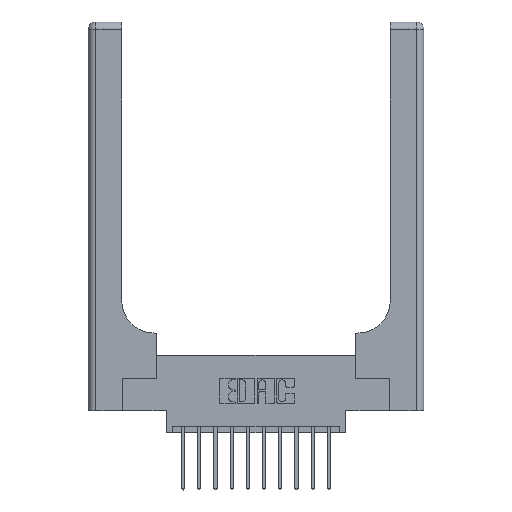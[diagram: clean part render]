
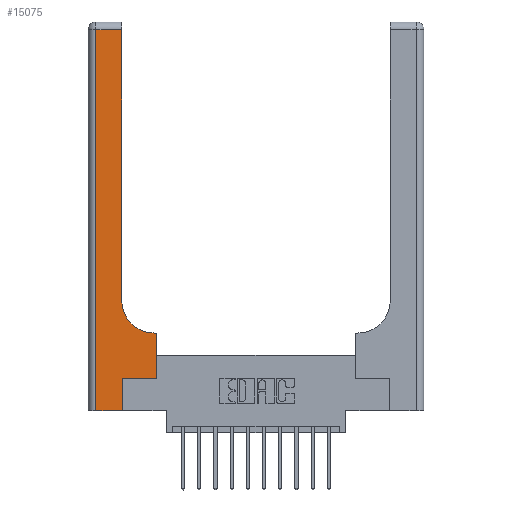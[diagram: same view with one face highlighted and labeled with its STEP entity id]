
A CAD part, top view. The second image highlights one B-rep face of the part: STEP entity #15075.
In plain terms, the highlighted planar face has unit normal (0, 0, 1).
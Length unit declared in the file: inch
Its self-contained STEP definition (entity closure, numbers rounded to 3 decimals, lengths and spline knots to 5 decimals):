
#54 = EDGE_CURVE ( 'NONE', #11182, #409, #9002, .T. ) ;
#239 = DIRECTION ( 'NONE',  ( 0., 0., -1. ) ) ;
#258 = DIRECTION ( 'NONE',  ( 0., 1., 0. ) ) ;
#409 = VERTEX_POINT ( 'NONE', #15262 ) ;
#423 = EDGE_CURVE ( 'NONE', #1495, #7632, #7598, .T. ) ;
#879 = DIRECTION ( 'NONE',  ( -1., 0., 0. ) ) ;
#1193 = ORIENTED_EDGE ( 'NONE', *, *, #54, .T. ) ;
#1268 = LINE ( 'NONE', #7843, #14576 ) ;
#1495 = VERTEX_POINT ( 'NONE', #8806 ) ;
#1577 = CARTESIAN_POINT ( 'NONE',  ( 0.26, 3., 0.37 ) ) ;
#1622 = DIRECTION ( 'NONE',  ( 0., -1., 0. ) ) ;
#1804 = DIRECTION ( 'NONE',  ( 1., 0., 0. ) ) ;
#2093 = ORIENTED_EDGE ( 'NONE', *, *, #2830, .T. ) ;
#2153 = CARTESIAN_POINT ( 'NONE',  ( 0., 2.94, 0.37 ) ) ;
#2456 = EDGE_LOOP ( 'NONE', ( #12871, #12136, #6369, #4838, #4947, #2093, #2734, #1193, #13378 ) ) ;
#2734 = ORIENTED_EDGE ( 'NONE', *, *, #3348, .T. ) ;
#2746 = EDGE_CURVE ( 'NONE', #15318, #7378, #5762, .T. ) ;
#2830 = EDGE_CURVE ( 'NONE', #7632, #5285, #5391, .T. ) ;
#2874 = CARTESIAN_POINT ( 'NONE',  ( 0.06, 3., 0.37 ) ) ;
#3275 = CARTESIAN_POINT ( 'NONE',  ( 0.265, 0.25, 0.37 ) ) ;
#3348 = EDGE_CURVE ( 'NONE', #5285, #11182, #1268, .T. ) ;
#3656 = EDGE_CURVE ( 'NONE', #14289, #15318, #6920, .T. ) ;
#4657 = VECTOR ( 'NONE', #258, 39.37008 ) ;
#4838 = ORIENTED_EDGE ( 'NONE', *, *, #12543, .T. ) ;
#4947 = ORIENTED_EDGE ( 'NONE', *, *, #423, .T. ) ;
#5273 = VECTOR ( 'NONE', #7014, 39.37008 ) ;
#5285 = VERTEX_POINT ( 'NONE', #15860 ) ;
#5391 = LINE ( 'NONE', #11786, #7926 ) ;
#5394 = CARTESIAN_POINT ( 'NONE',  ( 0., 0., 0.37 ) ) ;
#5567 = VECTOR ( 'NONE', #12917, 39.37008 ) ;
#5762 = LINE ( 'NONE', #2874, #12457 ) ;
#5952 = LINE ( 'NONE', #5394, #5567 ) ;
#6024 = CARTESIAN_POINT ( 'NONE',  ( 0.528, 0.6, 0.37 ) ) ;
#6028 = CARTESIAN_POINT ( 'NONE',  ( 0.26, 0.85, 0.37 ) ) ;
#6369 = ORIENTED_EDGE ( 'NONE', *, *, #2746, .T. ) ;
#6869 = EDGE_CURVE ( 'NONE', #12926, #14289, #14419, .T. ) ;
#6901 = CARTESIAN_POINT ( 'NONE',  ( 0.06, 2.94, 0.37 ) ) ;
#6920 = LINE ( 'NONE', #2153, #9893 ) ;
#7014 = DIRECTION ( 'NONE',  ( -1., 0., 0. ) ) ;
#7131 = CARTESIAN_POINT ( 'NONE',  ( 0.51, 0.85, 0.37 ) ) ;
#7142 = EDGE_CURVE ( 'NONE', #409, #12926, #13857, .T. ) ;
#7378 = VERTEX_POINT ( 'NONE', #10061 ) ;
#7598 = LINE ( 'NONE', #12763, #4657 ) ;
#7632 = VERTEX_POINT ( 'NONE', #3275 ) ;
#7676 = CARTESIAN_POINT ( 'NONE',  ( 0.26, 0.6, 0.37 ) ) ;
#7722 = PLANE ( 'NONE',  #10926 ) ;
#7843 = CARTESIAN_POINT ( 'NONE',  ( 0.528, 0.25, 0.37 ) ) ;
#7926 = VECTOR ( 'NONE', #1804, 39.37008 ) ;
#8026 = FACE_OUTER_BOUND ( 'NONE', #2456, .T. ) ;
#8381 = DIRECTION ( 'NONE',  ( 1., 0., 0. ) ) ;
#8806 = CARTESIAN_POINT ( 'NONE',  ( 0.265, 0., 0.37 ) ) ;
#8997 = DIRECTION ( 'NONE',  ( -1., 0., 0. ) ) ;
#9002 = LINE ( 'NONE', #7676, #5273 ) ;
#9112 = DIRECTION ( 'NONE',  ( 0., 1., 0. ) ) ;
#9893 = VECTOR ( 'NONE', #879, 39.37008 ) ;
#10061 = CARTESIAN_POINT ( 'NONE',  ( 0.06, 0., 0.37 ) ) ;
#10926 = AXIS2_PLACEMENT_3D ( 'NONE', #11479, #239, #8997 ) ;
#11182 = VERTEX_POINT ( 'NONE', #6024 ) ;
#11479 = CARTESIAN_POINT ( 'NONE',  ( 0., 3., 0.37 ) ) ;
#11786 = CARTESIAN_POINT ( 'NONE',  ( 0.265, 0.25, 0.37 ) ) ;
#12136 = ORIENTED_EDGE ( 'NONE', *, *, #3656, .T. ) ;
#12375 = CARTESIAN_POINT ( 'NONE',  ( 0.26, 2.94, 0.37 ) ) ;
#12457 = VECTOR ( 'NONE', #1622, 39.37008 ) ;
#12543 = EDGE_CURVE ( 'NONE', #7378, #1495, #5952, .T. ) ;
#12763 = CARTESIAN_POINT ( 'NONE',  ( 0.265, 0., 0.37 ) ) ;
#12871 = ORIENTED_EDGE ( 'NONE', *, *, #6869, .T. ) ;
#12917 = DIRECTION ( 'NONE',  ( 1., 0., 0. ) ) ;
#12926 = VERTEX_POINT ( 'NONE', #6028 ) ;
#13376 = AXIS2_PLACEMENT_3D ( 'NONE', #7131, #15865, #8381 ) ;
#13378 = ORIENTED_EDGE ( 'NONE', *, *, #7142, .T. ) ;
#13857 = CIRCLE ( 'NONE', #13376, 0.25 ) ;
#14047 = VECTOR ( 'NONE', #15313, 39.37008 ) ;
#14289 = VERTEX_POINT ( 'NONE', #12375 ) ;
#14419 = LINE ( 'NONE', #1577, #14047 ) ;
#14576 = VECTOR ( 'NONE', #9112, 39.37008 ) ;
#15075 = ADVANCED_FACE ( 'NONE', ( #8026 ), #7722, .F. ) ;
#15262 = CARTESIAN_POINT ( 'NONE',  ( 0.51, 0.6, 0.37 ) ) ;
#15313 = DIRECTION ( 'NONE',  ( 0., 1., 0. ) ) ;
#15318 = VERTEX_POINT ( 'NONE', #6901 ) ;
#15860 = CARTESIAN_POINT ( 'NONE',  ( 0.528, 0.25, 0.37 ) ) ;
#15865 = DIRECTION ( 'NONE',  ( 0., 0., -1. ) ) ;
